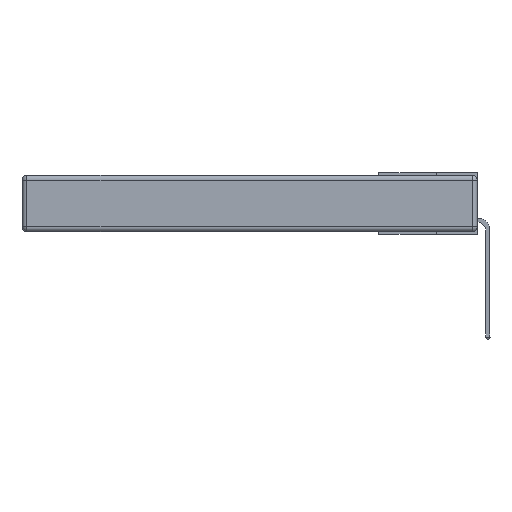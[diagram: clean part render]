
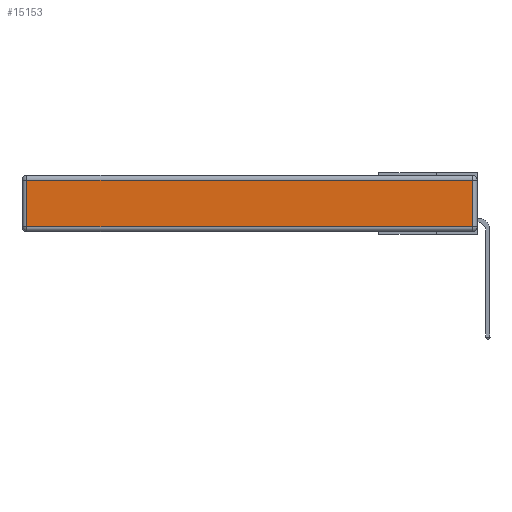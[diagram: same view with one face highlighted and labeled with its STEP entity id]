
A CAD part, left-side view. The second image highlights one B-rep face of the part: STEP entity #15153.
In plain terms, the highlighted planar face has unit normal (-1, 0, 0).
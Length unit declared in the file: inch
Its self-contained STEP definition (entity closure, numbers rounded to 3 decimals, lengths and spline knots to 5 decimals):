
#203 = ORIENTED_EDGE ( 'NONE', *, *, #9742, .T. ) ;
#1643 = LINE ( 'NONE', #21909, #10772 ) ;
#2118 = VERTEX_POINT ( 'NONE', #5971 ) ;
#2341 = EDGE_CURVE ( 'NONE', #2417, #2118, #8617, .T. ) ;
#2417 = VERTEX_POINT ( 'NONE', #18919 ) ;
#2625 = LINE ( 'NONE', #9466, #16894 ) ;
#3678 = CARTESIAN_POINT ( 'NONE',  ( 0., 0.03, -0.343 ) ) ;
#4423 = CARTESIAN_POINT ( 'NONE',  ( 0., 0., -0.343 ) ) ;
#4750 = DIRECTION ( 'NONE',  ( -1., 0., 0. ) ) ;
#5946 = AXIS2_PLACEMENT_3D ( 'NONE', #4423, #4750, #15599 ) ;
#5971 = CARTESIAN_POINT ( 'NONE',  ( 0., 2.72, -0.313 ) ) ;
#6602 = CARTESIAN_POINT ( 'NONE',  ( 0., 0.03, -0.03 ) ) ;
#7534 = EDGE_CURVE ( 'NONE', #2118, #20463, #2625, .T. ) ;
#8617 = LINE ( 'NONE', #18467, #15211 ) ;
#9297 = DIRECTION ( 'NONE',  ( 0., 0., -1. ) ) ;
#9466 = CARTESIAN_POINT ( 'NONE',  ( 0., 0., -0.313 ) ) ;
#9742 = EDGE_CURVE ( 'NONE', #20463, #14721, #17642, .T. ) ;
#9917 = FACE_OUTER_BOUND ( 'NONE', #13529, .T. ) ;
#10272 = ORIENTED_EDGE ( 'NONE', *, *, #7534, .T. ) ;
#10772 = VECTOR ( 'NONE', #12796, 39.37008 ) ;
#11975 = EDGE_CURVE ( 'NONE', #14721, #2417, #1643, .T. ) ;
#12747 = ORIENTED_EDGE ( 'NONE', *, *, #2341, .T. ) ;
#12796 = DIRECTION ( 'NONE',  ( 0., 1., 0. ) ) ;
#13529 = EDGE_LOOP ( 'NONE', ( #10272, #203, #14646, #12747 ) ) ;
#14646 = ORIENTED_EDGE ( 'NONE', *, *, #11975, .T. ) ;
#14721 = VERTEX_POINT ( 'NONE', #6602 ) ;
#15153 = ADVANCED_FACE ( 'NONE', ( #9917 ), #22928, .T. ) ;
#15211 = VECTOR ( 'NONE', #9297, 39.37008 ) ;
#15599 = DIRECTION ( 'NONE',  ( 0., 0., 1. ) ) ;
#16894 = VECTOR ( 'NONE', #22274, 39.37008 ) ;
#17642 = LINE ( 'NONE', #3678, #22248 ) ;
#18467 = CARTESIAN_POINT ( 'NONE',  ( 0., 2.72, -0.343 ) ) ;
#18660 = CARTESIAN_POINT ( 'NONE',  ( 0., 0.03, -0.313 ) ) ;
#18919 = CARTESIAN_POINT ( 'NONE',  ( 0., 2.72, -0.03 ) ) ;
#20463 = VERTEX_POINT ( 'NONE', #18660 ) ;
#21909 = CARTESIAN_POINT ( 'NONE',  ( 0., 2.75, -0.03 ) ) ;
#22248 = VECTOR ( 'NONE', #23612, 39.37008 ) ;
#22274 = DIRECTION ( 'NONE',  ( 0., -1., 0. ) ) ;
#22928 = PLANE ( 'NONE',  #5946 ) ;
#23612 = DIRECTION ( 'NONE',  ( 0., 0., 1. ) ) ;
